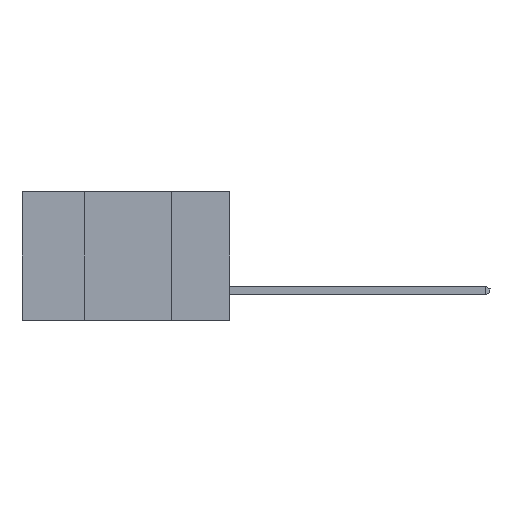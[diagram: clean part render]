
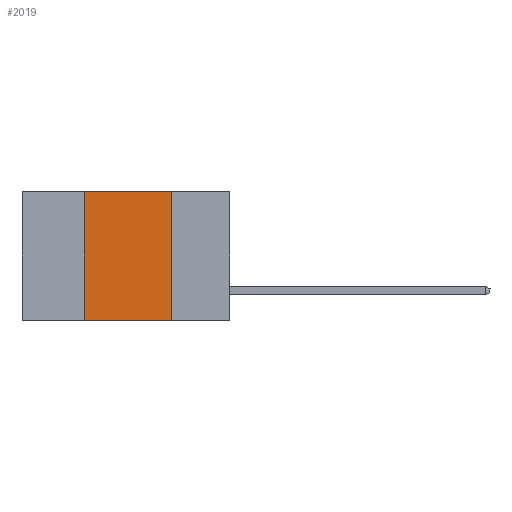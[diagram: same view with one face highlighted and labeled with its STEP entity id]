
A CAD part, left-side view. The second image highlights one B-rep face of the part: STEP entity #2019.
In plain terms, the highlighted planar face has unit normal (-1, 0, 0).
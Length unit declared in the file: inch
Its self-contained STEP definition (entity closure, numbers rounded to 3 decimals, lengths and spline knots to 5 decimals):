
#84 = CARTESIAN_POINT ( 'NONE',  ( 0., 0.17, 0. ) ) ;
#300 = EDGE_CURVE ( 'NONE', #6882, #5359, #12924, .T. ) ;
#530 = CARTESIAN_POINT ( 'NONE',  ( 0., 0.6, 0. ) ) ;
#925 = VERTEX_POINT ( 'NONE', #12410 ) ;
#1090 = CARTESIAN_POINT ( 'NONE',  ( 0., 0.42, -0.37 ) ) ;
#2019 = ADVANCED_FACE ( 'NONE', ( #9968 ), #6273, .F. ) ;
#3187 = LINE ( 'NONE', #9113, #15095 ) ;
#4133 = DIRECTION ( 'NONE',  ( 0., 0., -1. ) ) ;
#4513 = CARTESIAN_POINT ( 'NONE',  ( 0., 0.17, -0.37 ) ) ;
#5359 = VERTEX_POINT ( 'NONE', #4513 ) ;
#6273 = PLANE ( 'NONE',  #8799 ) ;
#6472 = ORIENTED_EDGE ( 'NONE', *, *, #300, .F. ) ;
#6606 = LINE ( 'NONE', #530, #11833 ) ;
#6882 = VERTEX_POINT ( 'NONE', #84 ) ;
#6971 = DIRECTION ( 'NONE',  ( 0., 0., 1. ) ) ;
#7040 = DIRECTION ( 'NONE',  ( 0., 0., -1. ) ) ;
#7181 = EDGE_CURVE ( 'NONE', #8027, #925, #12846, .T. ) ;
#7878 = DIRECTION ( 'NONE',  ( 0., -1., 0. ) ) ;
#7972 = ORIENTED_EDGE ( 'NONE', *, *, #7181, .F. ) ;
#8027 = VERTEX_POINT ( 'NONE', #1090 ) ;
#8799 = AXIS2_PLACEMENT_3D ( 'NONE', #9822, #14536, #4133 ) ;
#9113 = CARTESIAN_POINT ( 'NONE',  ( 0., 0.6, -0.37 ) ) ;
#9543 = EDGE_CURVE ( 'NONE', #925, #6882, #6606, .T. ) ;
#9594 = VECTOR ( 'NONE', #6971, 39.37008 ) ;
#9822 = CARTESIAN_POINT ( 'NONE',  ( 0., 0.6, 0. ) ) ;
#9919 = ORIENTED_EDGE ( 'NONE', *, *, #14945, .T. ) ;
#9968 = FACE_OUTER_BOUND ( 'NONE', #12756, .T. ) ;
#10513 = CARTESIAN_POINT ( 'NONE',  ( 0., 0.17, -0.37 ) ) ;
#11672 = CARTESIAN_POINT ( 'NONE',  ( 0., 0.42, -0.37 ) ) ;
#11833 = VECTOR ( 'NONE', #12239, 39.37008 ) ;
#12239 = DIRECTION ( 'NONE',  ( 0., -1., 0. ) ) ;
#12410 = CARTESIAN_POINT ( 'NONE',  ( 0., 0.42, 0. ) ) ;
#12756 = EDGE_LOOP ( 'NONE', ( #6472, #12783, #7972, #9919 ) ) ;
#12783 = ORIENTED_EDGE ( 'NONE', *, *, #9543, .F. ) ;
#12846 = LINE ( 'NONE', #11672, #9594 ) ;
#12924 = LINE ( 'NONE', #10513, #14091 ) ;
#14091 = VECTOR ( 'NONE', #7040, 39.37008 ) ;
#14536 = DIRECTION ( 'NONE',  ( 1., 0., 0. ) ) ;
#14945 = EDGE_CURVE ( 'NONE', #8027, #5359, #3187, .T. ) ;
#15095 = VECTOR ( 'NONE', #7878, 39.37008 ) ;
